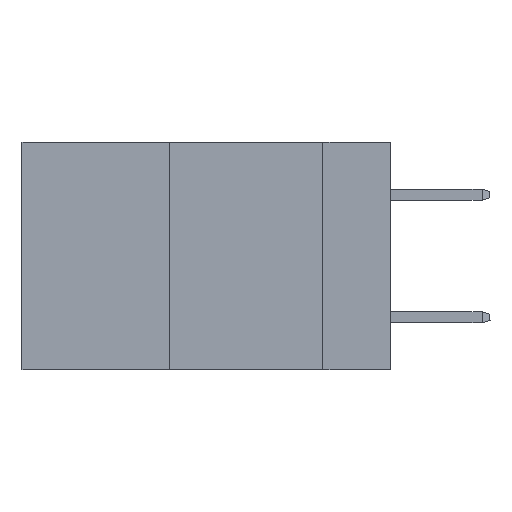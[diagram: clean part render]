
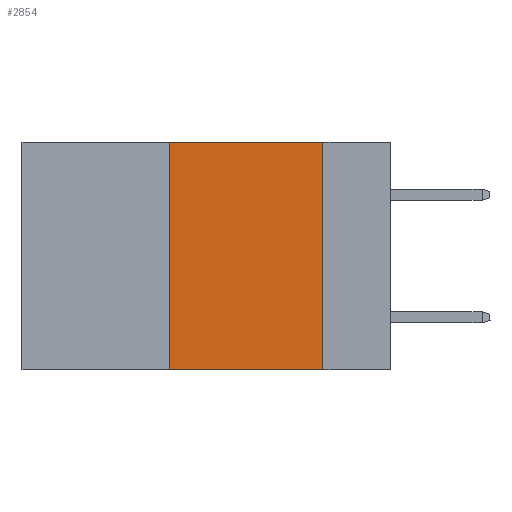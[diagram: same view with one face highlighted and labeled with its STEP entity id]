
A CAD part, left-side view. The second image highlights one B-rep face of the part: STEP entity #2854.
In plain terms, the highlighted planar face has unit normal (-1, 0, 0).
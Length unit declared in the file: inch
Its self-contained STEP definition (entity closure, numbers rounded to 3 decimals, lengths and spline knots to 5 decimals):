
#806 = EDGE_CURVE ( 'NONE', #10025, #3892, #12054, .T. ) ;
#2206 = ORIENTED_EDGE ( 'NONE', *, *, #806, .F. ) ;
#2703 = FACE_OUTER_BOUND ( 'NONE', #4467, .T. ) ;
#2776 = AXIS2_PLACEMENT_3D ( 'NONE', #9669, #8863, #11718 ) ;
#2854 = ADVANCED_FACE ( 'NONE', ( #2703 ), #5529, .F. ) ;
#2856 = EDGE_CURVE ( 'NONE', #10025, #5856, #10665, .T. ) ;
#3138 = EDGE_CURVE ( 'NONE', #3892, #5648, #9071, .T. ) ;
#3189 = CARTESIAN_POINT ( 'NONE',  ( 0., 0.11, 0. ) ) ;
#3294 = CARTESIAN_POINT ( 'NONE',  ( 0., 0.11, 0. ) ) ;
#3314 = CARTESIAN_POINT ( 'NONE',  ( 0., 0.36, 0. ) ) ;
#3653 = CARTESIAN_POINT ( 'NONE',  ( 0., 0.11, -0.37 ) ) ;
#3892 = VERTEX_POINT ( 'NONE', #3314 ) ;
#4088 = EDGE_CURVE ( 'NONE', #5648, #5856, #7920, .T. ) ;
#4425 = DIRECTION ( 'NONE',  ( 0., -1., 0. ) ) ;
#4467 = EDGE_LOOP ( 'NONE', ( #5213, #11968, #2206, #11694 ) ) ;
#4546 = CARTESIAN_POINT ( 'NONE',  ( 0., 0.6, 0. ) ) ;
#5213 = ORIENTED_EDGE ( 'NONE', *, *, #4088, .F. ) ;
#5529 = PLANE ( 'NONE',  #2776 ) ;
#5648 = VERTEX_POINT ( 'NONE', #3189 ) ;
#5746 = VECTOR ( 'NONE', #6143, 39.37008 ) ;
#5856 = VERTEX_POINT ( 'NONE', #3653 ) ;
#6143 = DIRECTION ( 'NONE',  ( 0., -1., 0. ) ) ;
#6591 = DIRECTION ( 'NONE',  ( 0., 0., -1. ) ) ;
#6938 = VECTOR ( 'NONE', #4425, 39.37008 ) ;
#7567 = CARTESIAN_POINT ( 'NONE',  ( 0., 0.36, -0.37 ) ) ;
#7736 = CARTESIAN_POINT ( 'NONE',  ( 0., 0.36, 0. ) ) ;
#7745 = DIRECTION ( 'NONE',  ( 0., 0., 1. ) ) ;
#7920 = LINE ( 'NONE', #3294, #10068 ) ;
#8863 = DIRECTION ( 'NONE',  ( 1., 0., 0. ) ) ;
#9071 = LINE ( 'NONE', #4546, #6938 ) ;
#9669 = CARTESIAN_POINT ( 'NONE',  ( 0., 0.6, 0. ) ) ;
#10025 = VERTEX_POINT ( 'NONE', #7567 ) ;
#10068 = VECTOR ( 'NONE', #6591, 39.37008 ) ;
#10224 = CARTESIAN_POINT ( 'NONE',  ( 0., 0.6, -0.37 ) ) ;
#10665 = LINE ( 'NONE', #10224, #5746 ) ;
#11694 = ORIENTED_EDGE ( 'NONE', *, *, #2856, .T. ) ;
#11718 = DIRECTION ( 'NONE',  ( 0., 0., -1. ) ) ;
#11791 = VECTOR ( 'NONE', #7745, 39.37008 ) ;
#11968 = ORIENTED_EDGE ( 'NONE', *, *, #3138, .F. ) ;
#12054 = LINE ( 'NONE', #7736, #11791 ) ;
